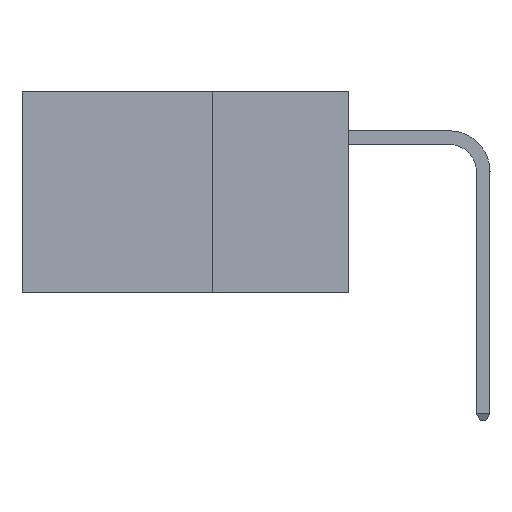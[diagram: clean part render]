
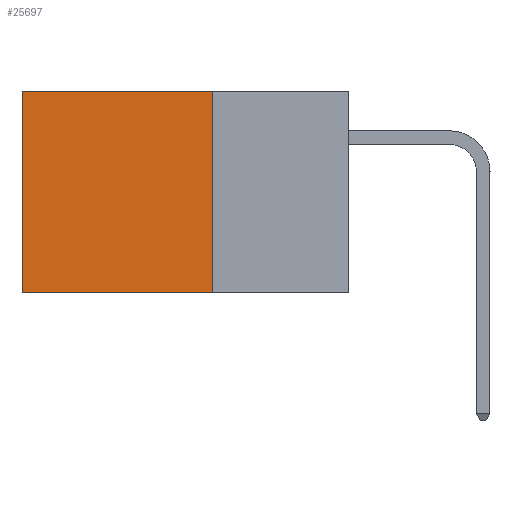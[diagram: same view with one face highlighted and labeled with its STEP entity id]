
A CAD part, left-side view. The second image highlights one B-rep face of the part: STEP entity #25697.
In plain terms, the highlighted planar face has unit normal (-1, 0, 0).
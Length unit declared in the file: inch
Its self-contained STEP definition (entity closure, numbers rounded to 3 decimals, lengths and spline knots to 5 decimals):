
#1656 = EDGE_CURVE ( 'NONE', #4932, #8935, #11470, .T. ) ;
#2642 = EDGE_CURVE ( 'NONE', #8935, #14674, #3436, .T. ) ;
#3243 = CARTESIAN_POINT ( 'NONE',  ( 0.2875, 0.25, 0. ) ) ;
#3436 = LINE ( 'NONE', #35385, #11957 ) ;
#4932 = VERTEX_POINT ( 'NONE', #34244 ) ;
#6623 = ORIENTED_EDGE ( 'NONE', *, *, #13449, .F. ) ;
#6704 = CARTESIAN_POINT ( 'NONE',  ( 0.2875, 0.25, 0. ) ) ;
#7276 = CARTESIAN_POINT ( 'NONE',  ( 0.2875, 0.25, 0. ) ) ;
#8883 = AXIS2_PLACEMENT_3D ( 'NONE', #6704, #13180, #35199 ) ;
#8935 = VERTEX_POINT ( 'NONE', #39986 ) ;
#9921 = PLANE ( 'NONE',  #8883 ) ;
#9949 = ORIENTED_EDGE ( 'NONE', *, *, #18341, .F. ) ;
#11470 = LINE ( 'NONE', #7276, #18978 ) ;
#11957 = VECTOR ( 'NONE', #22899, 39.37008 ) ;
#12340 = VECTOR ( 'NONE', #32099, 39.37008 ) ;
#12897 = DIRECTION ( 'NONE',  ( 0., 0., -1. ) ) ;
#13180 = DIRECTION ( 'NONE',  ( 1., 0., 0. ) ) ;
#13449 = EDGE_CURVE ( 'NONE', #33078, #14674, #37462, .T. ) ;
#14674 = VERTEX_POINT ( 'NONE', #18460 ) ;
#15239 = ORIENTED_EDGE ( 'NONE', *, *, #2642, .T. ) ;
#17040 = VECTOR ( 'NONE', #12897, 39.37008 ) ;
#18341 = EDGE_CURVE ( 'NONE', #4932, #33078, #32771, .T. ) ;
#18460 = CARTESIAN_POINT ( 'NONE',  ( 0.2875, 0.6, -0.37 ) ) ;
#18978 = VECTOR ( 'NONE', #26304, 39.37008 ) ;
#22899 = DIRECTION ( 'NONE',  ( 0., 0., -1. ) ) ;
#23506 = ORIENTED_EDGE ( 'NONE', *, *, #1656, .T. ) ;
#25697 = ADVANCED_FACE ( 'NONE', ( #32861 ), #9921, .F. ) ;
#26076 = EDGE_LOOP ( 'NONE', ( #15239, #6623, #9949, #23506 ) ) ;
#26304 = DIRECTION ( 'NONE',  ( 0., 1., 0. ) ) ;
#28936 = CARTESIAN_POINT ( 'NONE',  ( 0.2875, 0.25, -0.37 ) ) ;
#32099 = DIRECTION ( 'NONE',  ( 0., 1., 0. ) ) ;
#32771 = LINE ( 'NONE', #3243, #17040 ) ;
#32861 = FACE_OUTER_BOUND ( 'NONE', #26076, .T. ) ;
#33078 = VERTEX_POINT ( 'NONE', #33911 ) ;
#33911 = CARTESIAN_POINT ( 'NONE',  ( 0.2875, 0.25, -0.37 ) ) ;
#34244 = CARTESIAN_POINT ( 'NONE',  ( 0.2875, 0.25, 0. ) ) ;
#35199 = DIRECTION ( 'NONE',  ( 0., 0., -1. ) ) ;
#35385 = CARTESIAN_POINT ( 'NONE',  ( 0.2875, 0.6, 0. ) ) ;
#37462 = LINE ( 'NONE', #28936, #12340 ) ;
#39986 = CARTESIAN_POINT ( 'NONE',  ( 0.2875, 0.6, 0. ) ) ;
